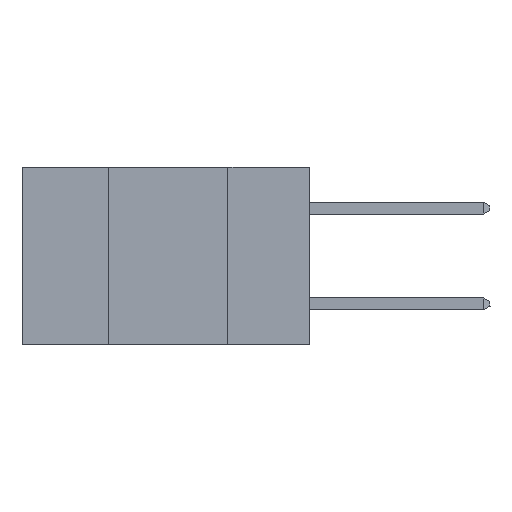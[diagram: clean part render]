
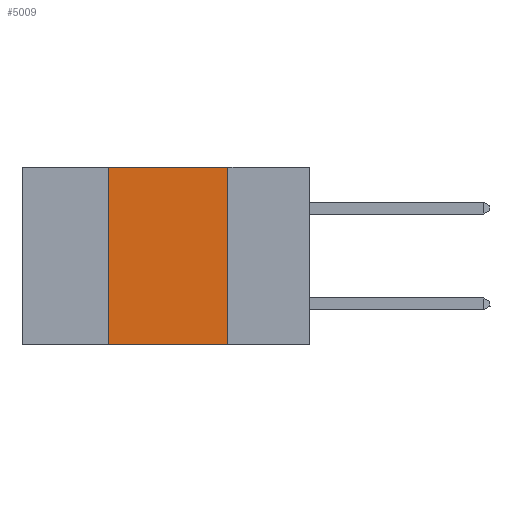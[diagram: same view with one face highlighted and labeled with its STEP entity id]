
A CAD part, left-side view. The second image highlights one B-rep face of the part: STEP entity #5009.
In plain terms, the highlighted planar face has unit normal (-1, 0, 0).
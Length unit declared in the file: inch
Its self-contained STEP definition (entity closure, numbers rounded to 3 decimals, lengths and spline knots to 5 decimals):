
#359 = EDGE_LOOP ( 'NONE', ( #697, #1061, #859, #1398 ) ) ;
#697 = ORIENTED_EDGE ( 'NONE', *, *, #19553, .F. ) ;
#743 = VECTOR ( 'NONE', #6258, 39.37008 ) ;
#859 = ORIENTED_EDGE ( 'NONE', *, *, #3292, .F. ) ;
#905 = DIRECTION ( 'NONE',  ( 0., -1., 0. ) ) ;
#1061 = ORIENTED_EDGE ( 'NONE', *, *, #2418, .F. ) ;
#1398 = ORIENTED_EDGE ( 'NONE', *, *, #6753, .T. ) ;
#2418 = EDGE_CURVE ( 'NONE', #3032, #15012, #14116, .T. ) ;
#2845 = DIRECTION ( 'NONE',  ( 0., 0., 1. ) ) ;
#3032 = VERTEX_POINT ( 'NONE', #5444 ) ;
#3292 = EDGE_CURVE ( 'NONE', #4158, #3032, #7390, .T. ) ;
#3549 = AXIS2_PLACEMENT_3D ( 'NONE', #20874, #18062, #21447 ) ;
#4125 = PLANE ( 'NONE',  #3549 ) ;
#4158 = VERTEX_POINT ( 'NONE', #15104 ) ;
#4521 = CARTESIAN_POINT ( 'NONE',  ( 0., 0.42, 0. ) ) ;
#4538 = CARTESIAN_POINT ( 'NONE',  ( 0., 0.6, -0.37 ) ) ;
#5009 = ADVANCED_FACE ( 'NONE', ( #9570 ), #4125, .F. ) ;
#5444 = CARTESIAN_POINT ( 'NONE',  ( 0., 0.42, 0. ) ) ;
#5879 = LINE ( 'NONE', #9189, #18783 ) ;
#6258 = DIRECTION ( 'NONE',  ( 0., -1., 0. ) ) ;
#6274 = VECTOR ( 'NONE', #2845, 39.37008 ) ;
#6753 = EDGE_CURVE ( 'NONE', #4158, #16891, #15521, .T. ) ;
#7390 = LINE ( 'NONE', #4521, #6274 ) ;
#9189 = CARTESIAN_POINT ( 'NONE',  ( 0., 0.17, 0. ) ) ;
#9570 = FACE_OUTER_BOUND ( 'NONE', #359, .T. ) ;
#10847 = DIRECTION ( 'NONE',  ( 0., 0., -1. ) ) ;
#12667 = CARTESIAN_POINT ( 'NONE',  ( 0., 0.6, 0. ) ) ;
#14116 = LINE ( 'NONE', #12667, #19740 ) ;
#15012 = VERTEX_POINT ( 'NONE', #19523 ) ;
#15104 = CARTESIAN_POINT ( 'NONE',  ( 0., 0.42, -0.37 ) ) ;
#15521 = LINE ( 'NONE', #4538, #743 ) ;
#16891 = VERTEX_POINT ( 'NONE', #21468 ) ;
#18062 = DIRECTION ( 'NONE',  ( 1., 0., 0. ) ) ;
#18783 = VECTOR ( 'NONE', #10847, 39.37008 ) ;
#19523 = CARTESIAN_POINT ( 'NONE',  ( 0., 0.17, 0. ) ) ;
#19553 = EDGE_CURVE ( 'NONE', #15012, #16891, #5879, .T. ) ;
#19740 = VECTOR ( 'NONE', #905, 39.37008 ) ;
#20874 = CARTESIAN_POINT ( 'NONE',  ( 0., 0.6, 0. ) ) ;
#21447 = DIRECTION ( 'NONE',  ( 0., 0., -1. ) ) ;
#21468 = CARTESIAN_POINT ( 'NONE',  ( 0., 0.17, -0.37 ) ) ;
